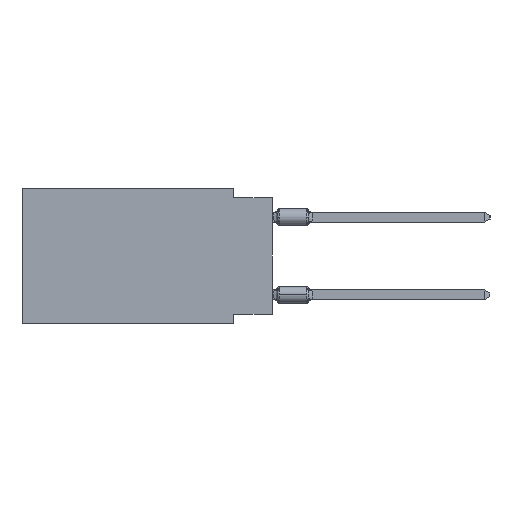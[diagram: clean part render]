
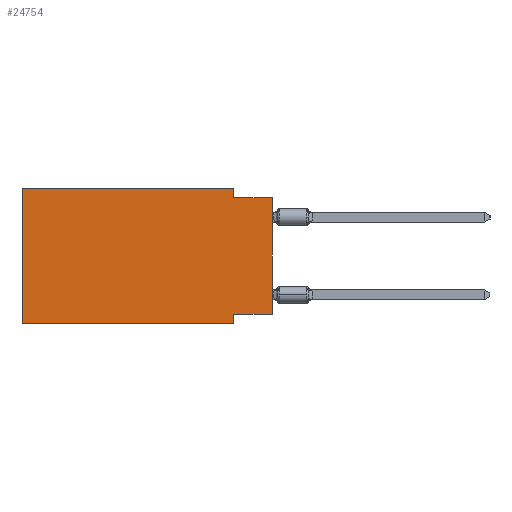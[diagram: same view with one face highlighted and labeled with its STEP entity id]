
A CAD part, left-side view. The second image highlights one B-rep face of the part: STEP entity #24754.
In plain terms, the highlighted planar face has unit normal (-1, 0, 0).
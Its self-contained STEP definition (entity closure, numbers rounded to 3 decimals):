
#36 = LINE ( 'NONE', #21947, #10274 ) ;
#276 = VECTOR ( 'NONE', #20429, 1000. ) ;
#535 = CARTESIAN_POINT ( 'NONE',  ( 0., 0., -8.255 ) ) ;
#756 = VECTOR ( 'NONE', #15302, 1000. ) ;
#1202 = EDGE_CURVE ( 'NONE', #9467, #22652, #20730, .T. ) ;
#1582 = DIRECTION ( 'NONE',  ( 0., -1., 0. ) ) ;
#1766 = CARTESIAN_POINT ( 'NONE',  ( 0., 2.54, 0. ) ) ;
#2110 = EDGE_CURVE ( 'NONE', #22652, #8330, #36, .T. ) ;
#2667 = EDGE_CURVE ( 'NONE', #12480, #22970, #17290, .T. ) ;
#2748 = CARTESIAN_POINT ( 'NONE',  ( 0., 16.383, 0. ) ) ;
#2860 = DIRECTION ( 'NONE',  ( 0., -1., 0. ) ) ;
#3393 = VECTOR ( 'NONE', #1582, 1000. ) ;
#3533 = CARTESIAN_POINT ( 'NONE',  ( 0., 2.54, -8.89 ) ) ;
#4340 = EDGE_CURVE ( 'NONE', #18891, #7956, #11678, .T. ) ;
#4669 = DIRECTION ( 'NONE',  ( 0., 1., 0. ) ) ;
#5128 = ORIENTED_EDGE ( 'NONE', *, *, #2110, .F. ) ;
#6357 = DIRECTION ( 'NONE',  ( 0., 0., -1. ) ) ;
#7208 = CARTESIAN_POINT ( 'NONE',  ( 0., 16.383, 0. ) ) ;
#7397 = CARTESIAN_POINT ( 'NONE',  ( 0., 0., 0. ) ) ;
#7423 = CARTESIAN_POINT ( 'NONE',  ( 0., 2.54, -0.635 ) ) ;
#7876 = LINE ( 'NONE', #1766, #22420 ) ;
#7935 = ORIENTED_EDGE ( 'NONE', *, *, #25348, .T. ) ;
#7956 = VERTEX_POINT ( 'NONE', #25760 ) ;
#7981 = CARTESIAN_POINT ( 'NONE',  ( 0., 2.54, 0. ) ) ;
#8330 = VERTEX_POINT ( 'NONE', #3533 ) ;
#8442 = VECTOR ( 'NONE', #13622, 1000. ) ;
#9350 = DIRECTION ( 'NONE',  ( 0., 0., -1. ) ) ;
#9369 = LINE ( 'NONE', #21051, #22217 ) ;
#9467 = VERTEX_POINT ( 'NONE', #23209 ) ;
#10217 = DIRECTION ( 'NONE',  ( 1., 0., 0. ) ) ;
#10274 = VECTOR ( 'NONE', #11866, 1000. ) ;
#10595 = LINE ( 'NONE', #2748, #276 ) ;
#10663 = CARTESIAN_POINT ( 'NONE',  ( 0., 16.383, 0. ) ) ;
#11075 = EDGE_CURVE ( 'NONE', #22970, #18891, #7876, .T. ) ;
#11678 = LINE ( 'NONE', #19787, #3393 ) ;
#11866 = DIRECTION ( 'NONE',  ( 0., 0., -1. ) ) ;
#12194 = CARTESIAN_POINT ( 'NONE',  ( 0., 16.383, 0. ) ) ;
#12480 = VERTEX_POINT ( 'NONE', #10663 ) ;
#13622 = DIRECTION ( 'NONE',  ( 0., 0., 1. ) ) ;
#14015 = AXIS2_PLACEMENT_3D ( 'NONE', #12194, #10217, #6357 ) ;
#14188 = FACE_OUTER_BOUND ( 'NONE', #15355, .T. ) ;
#14774 = CARTESIAN_POINT ( 'NONE',  ( 0., 2.54, -8.255 ) ) ;
#14831 = VERTEX_POINT ( 'NONE', #24301 ) ;
#15238 = ORIENTED_EDGE ( 'NONE', *, *, #4340, .F. ) ;
#15302 = DIRECTION ( 'NONE',  ( 0., -1., 0. ) ) ;
#15355 = EDGE_LOOP ( 'NONE', ( #24585, #15238, #23223, #24679, #23095, #7935, #5128, #20920 ) ) ;
#15755 = LINE ( 'NONE', #7397, #8442 ) ;
#17290 = LINE ( 'NONE', #7208, #756 ) ;
#18891 = VERTEX_POINT ( 'NONE', #7423 ) ;
#19196 = EDGE_CURVE ( 'NONE', #14831, #12480, #10595, .T. ) ;
#19787 = CARTESIAN_POINT ( 'NONE',  ( 0., 0., -0.635 ) ) ;
#20429 = DIRECTION ( 'NONE',  ( 0., 0., 1. ) ) ;
#20730 = LINE ( 'NONE', #535, #23437 ) ;
#20920 = ORIENTED_EDGE ( 'NONE', *, *, #1202, .F. ) ;
#21051 = CARTESIAN_POINT ( 'NONE',  ( 0., 16.383, -8.89 ) ) ;
#21947 = CARTESIAN_POINT ( 'NONE',  ( 0., 2.54, -8.89 ) ) ;
#22009 = EDGE_CURVE ( 'NONE', #9467, #7956, #15755, .T. ) ;
#22217 = VECTOR ( 'NONE', #2860, 1000. ) ;
#22286 = PLANE ( 'NONE',  #14015 ) ;
#22420 = VECTOR ( 'NONE', #9350, 1000. ) ;
#22652 = VERTEX_POINT ( 'NONE', #14774 ) ;
#22970 = VERTEX_POINT ( 'NONE', #7981 ) ;
#23095 = ORIENTED_EDGE ( 'NONE', *, *, #19196, .F. ) ;
#23209 = CARTESIAN_POINT ( 'NONE',  ( 0., 0., -8.255 ) ) ;
#23223 = ORIENTED_EDGE ( 'NONE', *, *, #11075, .F. ) ;
#23437 = VECTOR ( 'NONE', #4669, 1000. ) ;
#24301 = CARTESIAN_POINT ( 'NONE',  ( 0., 16.383, -8.89 ) ) ;
#24585 = ORIENTED_EDGE ( 'NONE', *, *, #22009, .T. ) ;
#24679 = ORIENTED_EDGE ( 'NONE', *, *, #2667, .F. ) ;
#24754 = ADVANCED_FACE ( 'NONE', ( #14188 ), #22286, .F. ) ;
#25348 = EDGE_CURVE ( 'NONE', #14831, #8330, #9369, .T. ) ;
#25760 = CARTESIAN_POINT ( 'NONE',  ( 0., 0., -0.635 ) ) ;
